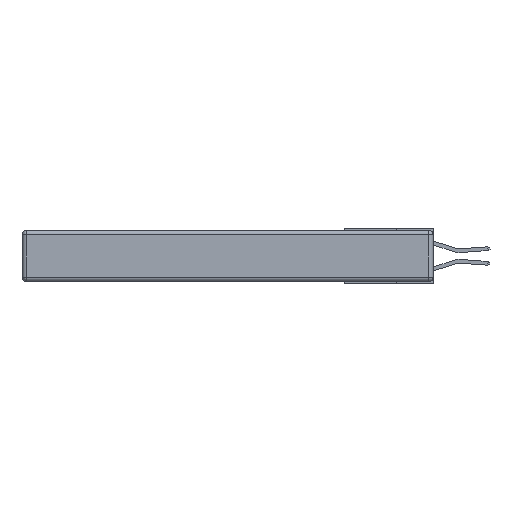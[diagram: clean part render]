
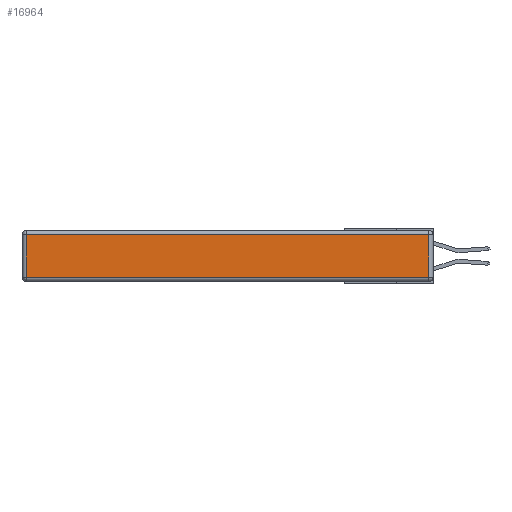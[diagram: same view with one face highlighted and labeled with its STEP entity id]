
A CAD part, left-side view. The second image highlights one B-rep face of the part: STEP entity #16964.
In plain terms, the highlighted planar face has unit normal (-1, 0, 0).
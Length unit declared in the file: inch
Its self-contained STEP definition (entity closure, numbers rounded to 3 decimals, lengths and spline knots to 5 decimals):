
#1282 = CARTESIAN_POINT ( 'NONE',  ( 0., 0., -0.343 ) ) ;
#2470 = ORIENTED_EDGE ( 'NONE', *, *, #10094, .T. ) ;
#3671 = DIRECTION ( 'NONE',  ( 0., 0., 1. ) ) ;
#3808 = VERTEX_POINT ( 'NONE', #12242 ) ;
#4898 = LINE ( 'NONE', #19639, #23722 ) ;
#5668 = AXIS2_PLACEMENT_3D ( 'NONE', #1282, #19380, #13571 ) ;
#7096 = PLANE ( 'NONE',  #5668 ) ;
#9060 = LINE ( 'NONE', #12687, #13522 ) ;
#9960 = ORIENTED_EDGE ( 'NONE', *, *, #22124, .T. ) ;
#10094 = EDGE_CURVE ( 'NONE', #3808, #15554, #22700, .T. ) ;
#11606 = ORIENTED_EDGE ( 'NONE', *, *, #13303, .T. ) ;
#12242 = CARTESIAN_POINT ( 'NONE',  ( 0., 0.03, -0.03 ) ) ;
#12493 = VECTOR ( 'NONE', #13505, 39.37008 ) ;
#12589 = FACE_OUTER_BOUND ( 'NONE', #13384, .T. ) ;
#12687 = CARTESIAN_POINT ( 'NONE',  ( 0., 2.72, -0.343 ) ) ;
#13250 = VECTOR ( 'NONE', #26381, 39.37008 ) ;
#13303 = EDGE_CURVE ( 'NONE', #14458, #20027, #13901, .T. ) ;
#13384 = EDGE_LOOP ( 'NONE', ( #11606, #9960, #2470, #19622 ) ) ;
#13413 = CARTESIAN_POINT ( 'NONE',  ( 0., 2.75, -0.03 ) ) ;
#13505 = DIRECTION ( 'NONE',  ( 0., 1., 0. ) ) ;
#13522 = VECTOR ( 'NONE', #20811, 39.37008 ) ;
#13571 = DIRECTION ( 'NONE',  ( 0., 0., 1. ) ) ;
#13901 = LINE ( 'NONE', #20501, #13250 ) ;
#14154 = CARTESIAN_POINT ( 'NONE',  ( 0., 2.72, -0.313 ) ) ;
#14458 = VERTEX_POINT ( 'NONE', #14154 ) ;
#15538 = CARTESIAN_POINT ( 'NONE',  ( 0., 0.03, -0.313 ) ) ;
#15554 = VERTEX_POINT ( 'NONE', #23777 ) ;
#16964 = ADVANCED_FACE ( 'NONE', ( #12589 ), #7096, .T. ) ;
#17191 = EDGE_CURVE ( 'NONE', #15554, #14458, #9060, .T. ) ;
#19380 = DIRECTION ( 'NONE',  ( -1., 0., 0. ) ) ;
#19622 = ORIENTED_EDGE ( 'NONE', *, *, #17191, .T. ) ;
#19639 = CARTESIAN_POINT ( 'NONE',  ( 0., 0.03, -0.343 ) ) ;
#20027 = VERTEX_POINT ( 'NONE', #15538 ) ;
#20501 = CARTESIAN_POINT ( 'NONE',  ( 0., 0., -0.313 ) ) ;
#20811 = DIRECTION ( 'NONE',  ( 0., 0., -1. ) ) ;
#22124 = EDGE_CURVE ( 'NONE', #20027, #3808, #4898, .T. ) ;
#22700 = LINE ( 'NONE', #13413, #12493 ) ;
#23722 = VECTOR ( 'NONE', #3671, 39.37008 ) ;
#23777 = CARTESIAN_POINT ( 'NONE',  ( 0., 2.72, -0.03 ) ) ;
#26381 = DIRECTION ( 'NONE',  ( 0., -1., 0. ) ) ;
